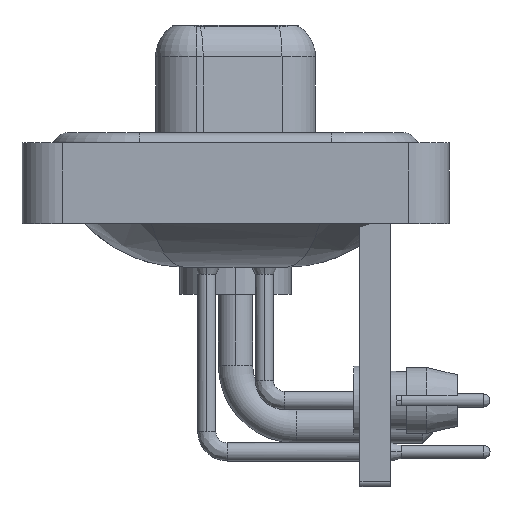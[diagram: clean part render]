
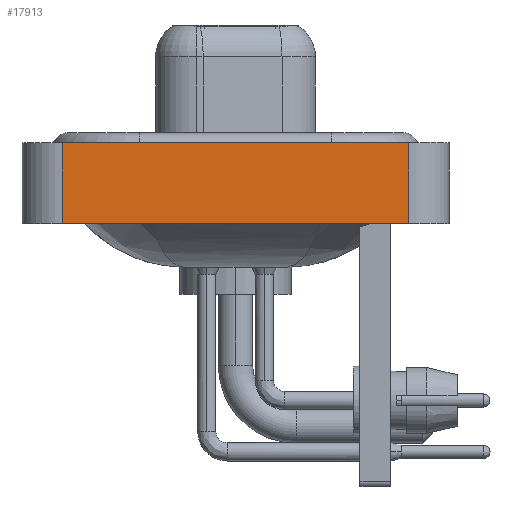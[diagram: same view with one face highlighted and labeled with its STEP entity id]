
A CAD part, left-side view. The second image highlights one B-rep face of the part: STEP entity #17913.
In plain terms, the highlighted planar face has unit normal (-1, 0, 0).
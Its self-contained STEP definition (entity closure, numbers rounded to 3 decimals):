
#522 = CARTESIAN_POINT ( 'NONE',  ( -7.25, 8.55, -3.6 ) ) ;
#2133 = VERTEX_POINT ( 'NONE', #7915 ) ;
#2878 = EDGE_CURVE ( 'NONE', #2133, #20703, #4239, .T. ) ;
#3171 = CARTESIAN_POINT ( 'NONE',  ( -7.25, -8.55, -3.6 ) ) ;
#3967 = CARTESIAN_POINT ( 'NONE',  ( -7.25, -8.55, 0.4 ) ) ;
#4053 = ORIENTED_EDGE ( 'NONE', *, *, #9178, .F. ) ;
#4239 = LINE ( 'NONE', #522, #7156 ) ;
#4263 = EDGE_LOOP ( 'NONE', ( #16835, #4053, #6809, #16967 ) ) ;
#4646 = LINE ( 'NONE', #7822, #18488 ) ;
#5543 = DIRECTION ( 'NONE',  ( -1., 0., 0. ) ) ;
#5647 = FACE_OUTER_BOUND ( 'NONE', #4263, .T. ) ;
#5780 = EDGE_CURVE ( 'NONE', #2133, #12575, #10298, .T. ) ;
#6809 = ORIENTED_EDGE ( 'NONE', *, *, #2878, .F. ) ;
#7156 = VECTOR ( 'NONE', #19817, 1000. ) ;
#7338 = AXIS2_PLACEMENT_3D ( 'NONE', #21345, #5543, #7570 ) ;
#7564 = EDGE_CURVE ( 'NONE', #12575, #20358, #4646, .T. ) ;
#7570 = DIRECTION ( 'NONE',  ( 0., 0., 1. ) ) ;
#7822 = CARTESIAN_POINT ( 'NONE',  ( -7.25, -8.55, -3.6 ) ) ;
#7915 = CARTESIAN_POINT ( 'NONE',  ( -7.25, 8.55, -3.6 ) ) ;
#9178 = EDGE_CURVE ( 'NONE', #20703, #20358, #19438, .T. ) ;
#9273 = PLANE ( 'NONE',  #7338 ) ;
#10298 = LINE ( 'NONE', #3171, #11245 ) ;
#11245 = VECTOR ( 'NONE', #17160, 1000. ) ;
#12575 = VERTEX_POINT ( 'NONE', #18251 ) ;
#13040 = CARTESIAN_POINT ( 'NONE',  ( -7.25, -8.55, 0.4 ) ) ;
#13817 = CARTESIAN_POINT ( 'NONE',  ( -7.25, 8.55, 0.4 ) ) ;
#16835 = ORIENTED_EDGE ( 'NONE', *, *, #7564, .T. ) ;
#16967 = ORIENTED_EDGE ( 'NONE', *, *, #5780, .T. ) ;
#17084 = VECTOR ( 'NONE', #17744, 1000. ) ;
#17160 = DIRECTION ( 'NONE',  ( 0., -1., 0. ) ) ;
#17744 = DIRECTION ( 'NONE',  ( 0., -1., 0. ) ) ;
#17913 = ADVANCED_FACE ( 'NONE', ( #5647 ), #9273, .T. ) ;
#18251 = CARTESIAN_POINT ( 'NONE',  ( -7.25, -8.55, -3.6 ) ) ;
#18488 = VECTOR ( 'NONE', #20338, 1000. ) ;
#19438 = LINE ( 'NONE', #3967, #17084 ) ;
#19817 = DIRECTION ( 'NONE',  ( 0., 0., 1. ) ) ;
#20338 = DIRECTION ( 'NONE',  ( 0., 0., 1. ) ) ;
#20358 = VERTEX_POINT ( 'NONE', #13040 ) ;
#20703 = VERTEX_POINT ( 'NONE', #13817 ) ;
#21345 = CARTESIAN_POINT ( 'NONE',  ( -7.25, -8.55, -3.6 ) ) ;
